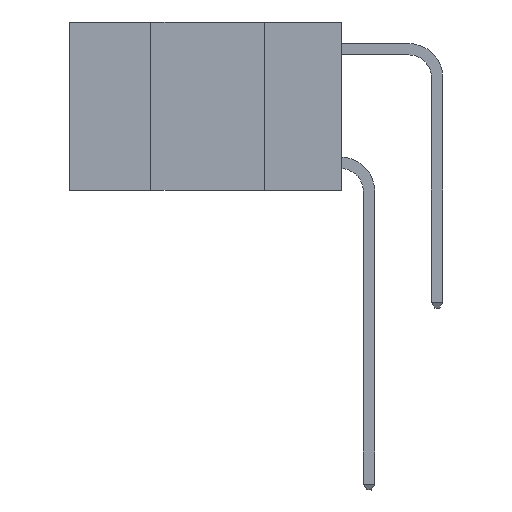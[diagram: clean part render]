
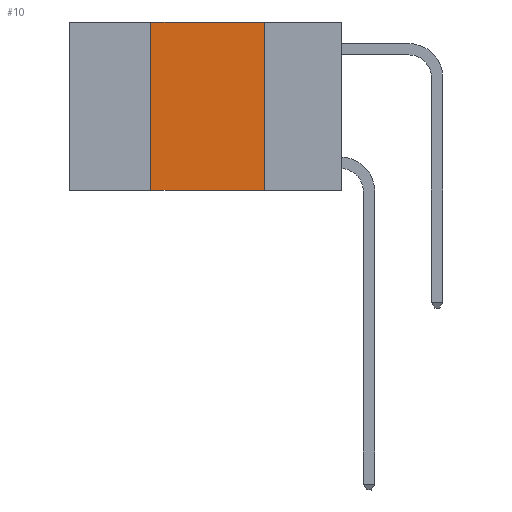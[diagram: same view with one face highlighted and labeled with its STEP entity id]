
A CAD part, left-side view. The second image highlights one B-rep face of the part: STEP entity #10.
In plain terms, the highlighted planar face has unit normal (-1, 0, 0).
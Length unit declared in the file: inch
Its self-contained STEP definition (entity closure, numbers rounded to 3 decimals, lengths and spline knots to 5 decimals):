
#10 = ADVANCED_FACE ( 'NONE', ( #5895 ), #8833, .F. ) ;
#750 = ORIENTED_EDGE ( 'NONE', *, *, #10890, .F. ) ;
#1081 = VECTOR ( 'NONE', #1397, 39.37008 ) ;
#1397 = DIRECTION ( 'NONE',  ( 0., 0., -1. ) ) ;
#2307 = DIRECTION ( 'NONE',  ( 1., 0., 0. ) ) ;
#2497 = CARTESIAN_POINT ( 'NONE',  ( 0., 0.17, -0.37 ) ) ;
#3226 = ORIENTED_EDGE ( 'NONE', *, *, #7051, .T. ) ;
#3829 = VERTEX_POINT ( 'NONE', #14759 ) ;
#4522 = CARTESIAN_POINT ( 'NONE',  ( 0., 0.6, 0. ) ) ;
#5819 = DIRECTION ( 'NONE',  ( 0., -1., 0. ) ) ;
#5895 = FACE_OUTER_BOUND ( 'NONE', #10457, .T. ) ;
#5955 = VERTEX_POINT ( 'NONE', #12953 ) ;
#6226 = DIRECTION ( 'NONE',  ( 0., 0., -1. ) ) ;
#6591 = LINE ( 'NONE', #4522, #13246 ) ;
#6936 = CARTESIAN_POINT ( 'NONE',  ( 0., 0.42, 0. ) ) ;
#7051 = EDGE_CURVE ( 'NONE', #3829, #9852, #11927, .T. ) ;
#7639 = LINE ( 'NONE', #9258, #1081 ) ;
#8142 = ORIENTED_EDGE ( 'NONE', *, *, #10164, .F. ) ;
#8449 = CARTESIAN_POINT ( 'NONE',  ( 0., 0.42, 0. ) ) ;
#8833 = PLANE ( 'NONE',  #14290 ) ;
#9258 = CARTESIAN_POINT ( 'NONE',  ( 0., 0.17, 0. ) ) ;
#9852 = VERTEX_POINT ( 'NONE', #2497 ) ;
#9915 = LINE ( 'NONE', #6936, #16539 ) ;
#10164 = EDGE_CURVE ( 'NONE', #3829, #15021, #9915, .T. ) ;
#10457 = EDGE_LOOP ( 'NONE', ( #16206, #750, #8142, #3226 ) ) ;
#10621 = EDGE_CURVE ( 'NONE', #5955, #9852, #7639, .T. ) ;
#10890 = EDGE_CURVE ( 'NONE', #15021, #5955, #6591, .T. ) ;
#11927 = LINE ( 'NONE', #12509, #15014 ) ;
#12279 = DIRECTION ( 'NONE',  ( 0., 0., 1. ) ) ;
#12509 = CARTESIAN_POINT ( 'NONE',  ( 0., 0.6, -0.37 ) ) ;
#12953 = CARTESIAN_POINT ( 'NONE',  ( 0., 0.17, 0. ) ) ;
#13246 = VECTOR ( 'NONE', #5819, 39.37008 ) ;
#14174 = CARTESIAN_POINT ( 'NONE',  ( 0., 0.6, 0. ) ) ;
#14290 = AXIS2_PLACEMENT_3D ( 'NONE', #14174, #2307, #6226 ) ;
#14759 = CARTESIAN_POINT ( 'NONE',  ( 0., 0.42, -0.37 ) ) ;
#15014 = VECTOR ( 'NONE', #16482, 39.37008 ) ;
#15021 = VERTEX_POINT ( 'NONE', #8449 ) ;
#16206 = ORIENTED_EDGE ( 'NONE', *, *, #10621, .F. ) ;
#16482 = DIRECTION ( 'NONE',  ( 0., -1., 0. ) ) ;
#16539 = VECTOR ( 'NONE', #12279, 39.37008 ) ;
